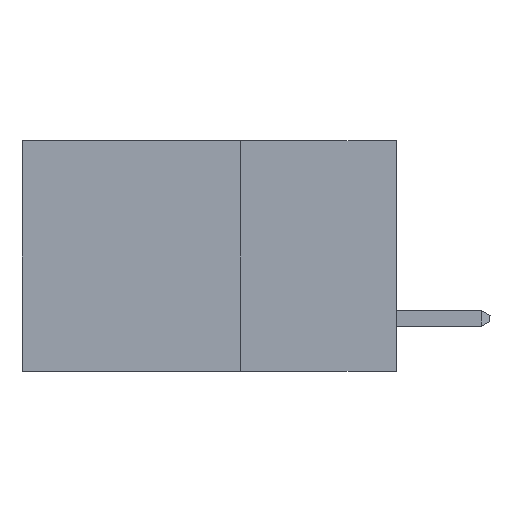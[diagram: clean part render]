
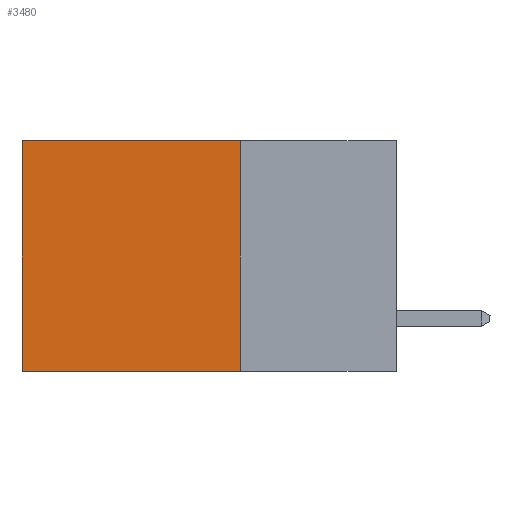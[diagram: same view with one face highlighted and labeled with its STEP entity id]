
A CAD part, left-side view. The second image highlights one B-rep face of the part: STEP entity #3480.
In plain terms, the highlighted planar face has unit normal (-1, 0, 0).
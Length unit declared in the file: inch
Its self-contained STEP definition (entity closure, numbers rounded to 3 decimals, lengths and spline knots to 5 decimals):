
#203 = DIRECTION ( 'NONE',  ( 0., 1., 0. ) ) ;
#236 = CARTESIAN_POINT ( 'NONE',  ( 0.2615, 0.6, -0.37 ) ) ;
#278 = VERTEX_POINT ( 'NONE', #8182 ) ;
#1062 = AXIS2_PLACEMENT_3D ( 'NONE', #9155, #9141, #9140 ) ;
#1277 = VECTOR ( 'NONE', #4819, 39.37008 ) ;
#1654 = EDGE_CURVE ( 'NONE', #278, #9103, #5724, .T. ) ;
#1961 = VERTEX_POINT ( 'NONE', #2050 ) ;
#1985 = VECTOR ( 'NONE', #203, 39.37008 ) ;
#2050 = CARTESIAN_POINT ( 'NONE',  ( 0.2615, 0.25, 0. ) ) ;
#2628 = LINE ( 'NONE', #9377, #6856 ) ;
#3347 = EDGE_LOOP ( 'NONE', ( #9252, #10037, #9927, #8623 ) ) ;
#3374 = DIRECTION ( 'NONE',  ( 0., 1., 0. ) ) ;
#3480 = ADVANCED_FACE ( 'NONE', ( #7162 ), #9217, .F. ) ;
#3486 = CARTESIAN_POINT ( 'NONE',  ( 0.2615, 0.25, 0. ) ) ;
#3999 = VERTEX_POINT ( 'NONE', #5909 ) ;
#4413 = EDGE_CURVE ( 'NONE', #1961, #278, #6859, .T. ) ;
#4819 = DIRECTION ( 'NONE',  ( 0., 0., -1. ) ) ;
#4884 = CARTESIAN_POINT ( 'NONE',  ( 0.2615, 0.6, -0.37 ) ) ;
#5724 = LINE ( 'NONE', #4884, #1277 ) ;
#5909 = CARTESIAN_POINT ( 'NONE',  ( 0.2615, 0.25, -0.37 ) ) ;
#6744 = EDGE_CURVE ( 'NONE', #3999, #9103, #8758, .T. ) ;
#6856 = VECTOR ( 'NONE', #8548, 39.37008 ) ;
#6859 = LINE ( 'NONE', #3486, #10804 ) ;
#7162 = FACE_OUTER_BOUND ( 'NONE', #3347, .T. ) ;
#8182 = CARTESIAN_POINT ( 'NONE',  ( 0.2615, 0.6, 0. ) ) ;
#8548 = DIRECTION ( 'NONE',  ( 0., 0., -1. ) ) ;
#8623 = ORIENTED_EDGE ( 'NONE', *, *, #4413, .T. ) ;
#8758 = LINE ( 'NONE', #10440, #1985 ) ;
#8918 = EDGE_CURVE ( 'NONE', #1961, #3999, #2628, .T. ) ;
#9103 = VERTEX_POINT ( 'NONE', #236 ) ;
#9140 = DIRECTION ( 'NONE',  ( 0., 0., -1. ) ) ;
#9141 = DIRECTION ( 'NONE',  ( 1., 0., 0. ) ) ;
#9155 = CARTESIAN_POINT ( 'NONE',  ( 0.2615, 0.25, -0.37 ) ) ;
#9217 = PLANE ( 'NONE',  #1062 ) ;
#9252 = ORIENTED_EDGE ( 'NONE', *, *, #1654, .T. ) ;
#9377 = CARTESIAN_POINT ( 'NONE',  ( 0.2615, 0.25, -0.37 ) ) ;
#9927 = ORIENTED_EDGE ( 'NONE', *, *, #8918, .F. ) ;
#10037 = ORIENTED_EDGE ( 'NONE', *, *, #6744, .F. ) ;
#10440 = CARTESIAN_POINT ( 'NONE',  ( 0.2615, 0.25, -0.37 ) ) ;
#10804 = VECTOR ( 'NONE', #3374, 39.37008 ) ;
